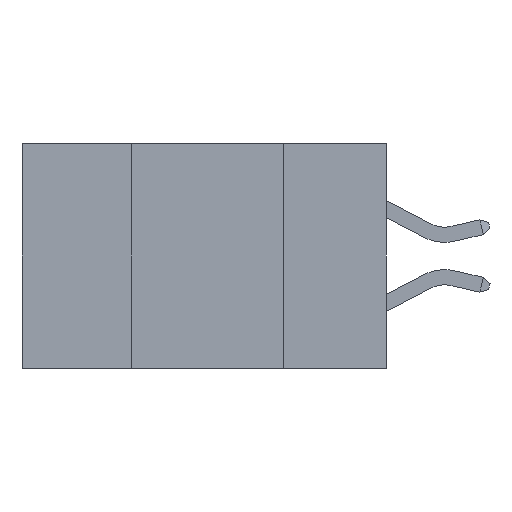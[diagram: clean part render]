
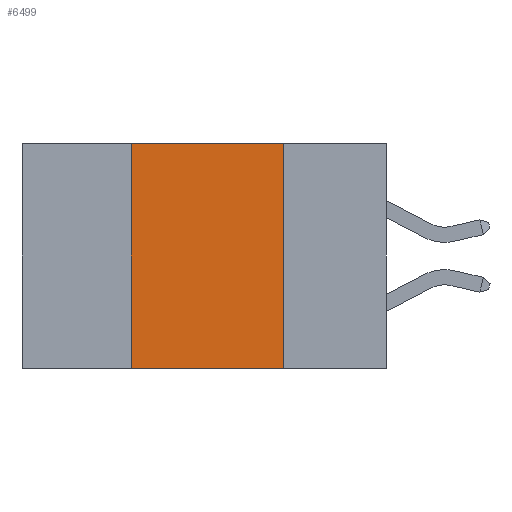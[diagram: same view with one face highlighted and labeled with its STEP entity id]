
A CAD part, left-side view. The second image highlights one B-rep face of the part: STEP entity #6499.
In plain terms, the highlighted planar face has unit normal (-1, 0, 0).
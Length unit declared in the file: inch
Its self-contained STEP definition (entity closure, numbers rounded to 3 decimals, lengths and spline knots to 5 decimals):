
#651 = VERTEX_POINT ( 'NONE', #2385 ) ;
#806 = DIRECTION ( 'NONE',  ( 0., -1., 0. ) ) ;
#912 = EDGE_LOOP ( 'NONE', ( #7914, #11243, #7464, #10807 ) ) ;
#1550 = EDGE_CURVE ( 'NONE', #5247, #17788, #4254, .T. ) ;
#1667 = DIRECTION ( 'NONE',  ( 0., 0., 1. ) ) ;
#2385 = CARTESIAN_POINT ( 'NONE',  ( 0., 0.17, 0. ) ) ;
#2575 = CARTESIAN_POINT ( 'NONE',  ( 0., 0.42, -0.37 ) ) ;
#2773 = LINE ( 'NONE', #5213, #16715 ) ;
#3032 = VERTEX_POINT ( 'NONE', #5327 ) ;
#3321 = LINE ( 'NONE', #10209, #10421 ) ;
#3965 = EDGE_CURVE ( 'NONE', #651, #3032, #5576, .T. ) ;
#4254 = LINE ( 'NONE', #12703, #11332 ) ;
#4546 = EDGE_CURVE ( 'NONE', #17788, #651, #3321, .T. ) ;
#5213 = CARTESIAN_POINT ( 'NONE',  ( 0., 0.6, -0.37 ) ) ;
#5247 = VERTEX_POINT ( 'NONE', #2575 ) ;
#5327 = CARTESIAN_POINT ( 'NONE',  ( 0., 0.17, -0.37 ) ) ;
#5576 = LINE ( 'NONE', #16102, #15791 ) ;
#6499 = ADVANCED_FACE ( 'NONE', ( #11692 ), #8703, .F. ) ;
#7243 = CARTESIAN_POINT ( 'NONE',  ( 0., 0.42, 0. ) ) ;
#7464 = ORIENTED_EDGE ( 'NONE', *, *, #1550, .F. ) ;
#7914 = ORIENTED_EDGE ( 'NONE', *, *, #3965, .F. ) ;
#8659 = DIRECTION ( 'NONE',  ( 0., 0., -1. ) ) ;
#8703 = PLANE ( 'NONE',  #17807 ) ;
#8849 = CARTESIAN_POINT ( 'NONE',  ( 0., 0.6, 0. ) ) ;
#9185 = DIRECTION ( 'NONE',  ( 1., 0., 0. ) ) ;
#10025 = DIRECTION ( 'NONE',  ( 0., -1., 0. ) ) ;
#10209 = CARTESIAN_POINT ( 'NONE',  ( 0., 0.6, 0. ) ) ;
#10421 = VECTOR ( 'NONE', #10025, 39.37008 ) ;
#10807 = ORIENTED_EDGE ( 'NONE', *, *, #12442, .T. ) ;
#11243 = ORIENTED_EDGE ( 'NONE', *, *, #4546, .F. ) ;
#11332 = VECTOR ( 'NONE', #1667, 39.37008 ) ;
#11692 = FACE_OUTER_BOUND ( 'NONE', #912, .T. ) ;
#12442 = EDGE_CURVE ( 'NONE', #5247, #3032, #2773, .T. ) ;
#12703 = CARTESIAN_POINT ( 'NONE',  ( 0., 0.42, -0.37 ) ) ;
#15791 = VECTOR ( 'NONE', #16156, 39.37008 ) ;
#16102 = CARTESIAN_POINT ( 'NONE',  ( 0., 0.17, -0.37 ) ) ;
#16156 = DIRECTION ( 'NONE',  ( 0., 0., -1. ) ) ;
#16715 = VECTOR ( 'NONE', #806, 39.37008 ) ;
#17788 = VERTEX_POINT ( 'NONE', #7243 ) ;
#17807 = AXIS2_PLACEMENT_3D ( 'NONE', #8849, #9185, #8659 ) ;
